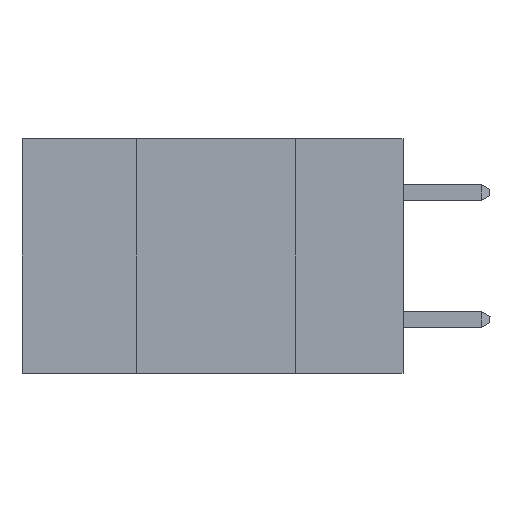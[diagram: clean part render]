
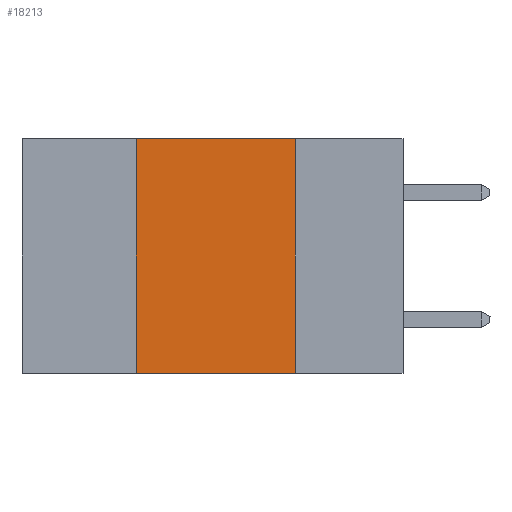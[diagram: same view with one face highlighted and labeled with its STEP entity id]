
A CAD part, left-side view. The second image highlights one B-rep face of the part: STEP entity #18213.
In plain terms, the highlighted planar face has unit normal (-1, 0, 0).
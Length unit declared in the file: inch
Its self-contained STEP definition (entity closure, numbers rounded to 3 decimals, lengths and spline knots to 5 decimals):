
#200 = VERTEX_POINT ( 'NONE', #2898 ) ;
#266 = LINE ( 'NONE', #39180, #39029 ) ;
#394 = DIRECTION ( 'NONE',  ( 0., -1., 0. ) ) ;
#857 = CARTESIAN_POINT ( 'NONE',  ( 0., 0.6, 0. ) ) ;
#2741 = ORIENTED_EDGE ( 'NONE', *, *, #26682, .F. ) ;
#2898 = CARTESIAN_POINT ( 'NONE',  ( 0., 0.42, -0.37 ) ) ;
#4824 = EDGE_CURVE ( 'NONE', #200, #34736, #19557, .T. ) ;
#5239 = EDGE_LOOP ( 'NONE', ( #25826, #2741, #40978, #33927 ) ) ;
#6143 = VECTOR ( 'NONE', #394, 39.37008 ) ;
#7928 = CARTESIAN_POINT ( 'NONE',  ( 0., 0.17, 0. ) ) ;
#7994 = LINE ( 'NONE', #40515, #14149 ) ;
#10472 = DIRECTION ( 'NONE',  ( 0., 0., 1. ) ) ;
#10881 = DIRECTION ( 'NONE',  ( 0., 0., -1. ) ) ;
#14057 = DIRECTION ( 'NONE',  ( 1., 0., 0. ) ) ;
#14149 = VECTOR ( 'NONE', #33723, 39.37008 ) ;
#16342 = CARTESIAN_POINT ( 'NONE',  ( 0., 0.17, -0.37 ) ) ;
#16493 = EDGE_CURVE ( 'NONE', #28284, #34736, #27297, .T. ) ;
#17925 = DIRECTION ( 'NONE',  ( 0., 0., -1. ) ) ;
#18213 = ADVANCED_FACE ( 'NONE', ( #33844 ), #30016, .F. ) ;
#19557 = LINE ( 'NONE', #19773, #6143 ) ;
#19773 = CARTESIAN_POINT ( 'NONE',  ( 0., 0.6, -0.37 ) ) ;
#20202 = CARTESIAN_POINT ( 'NONE',  ( 0., 0.42, 0. ) ) ;
#21319 = AXIS2_PLACEMENT_3D ( 'NONE', #857, #14057, #10881 ) ;
#25826 = ORIENTED_EDGE ( 'NONE', *, *, #16493, .F. ) ;
#26635 = VECTOR ( 'NONE', #17925, 39.37008 ) ;
#26682 = EDGE_CURVE ( 'NONE', #37822, #28284, #7994, .T. ) ;
#27297 = LINE ( 'NONE', #7928, #26635 ) ;
#28284 = VERTEX_POINT ( 'NONE', #29027 ) ;
#29027 = CARTESIAN_POINT ( 'NONE',  ( 0., 0.17, 0. ) ) ;
#30016 = PLANE ( 'NONE',  #21319 ) ;
#33723 = DIRECTION ( 'NONE',  ( 0., -1., 0. ) ) ;
#33844 = FACE_OUTER_BOUND ( 'NONE', #5239, .T. ) ;
#33927 = ORIENTED_EDGE ( 'NONE', *, *, #4824, .T. ) ;
#34736 = VERTEX_POINT ( 'NONE', #16342 ) ;
#37822 = VERTEX_POINT ( 'NONE', #20202 ) ;
#39029 = VECTOR ( 'NONE', #10472, 39.37008 ) ;
#39180 = CARTESIAN_POINT ( 'NONE',  ( 0., 0.42, 0. ) ) ;
#40465 = EDGE_CURVE ( 'NONE', #200, #37822, #266, .T. ) ;
#40515 = CARTESIAN_POINT ( 'NONE',  ( 0., 0.6, 0. ) ) ;
#40978 = ORIENTED_EDGE ( 'NONE', *, *, #40465, .F. ) ;
